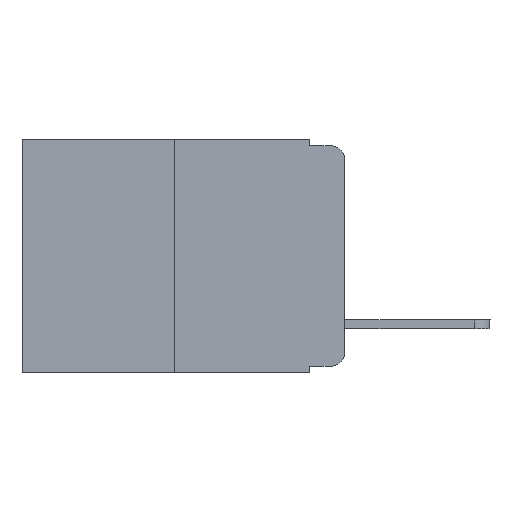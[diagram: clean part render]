
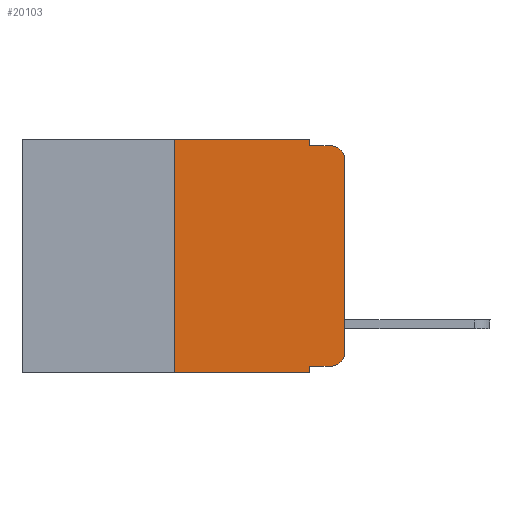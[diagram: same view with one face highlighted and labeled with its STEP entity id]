
A CAD part, left-side view. The second image highlights one B-rep face of the part: STEP entity #20103.
In plain terms, the highlighted planar face has unit normal (-1, 0, 0).
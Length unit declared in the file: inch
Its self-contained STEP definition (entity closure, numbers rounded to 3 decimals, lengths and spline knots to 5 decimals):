
#140 = LINE ( 'NONE', #18347, #10421 ) ;
#152 = CARTESIAN_POINT ( 'NONE',  ( 0., 0.02, -0.03 ) ) ;
#182 = DIRECTION ( 'NONE',  ( 0., 0., -1. ) ) ;
#248 = CARTESIAN_POINT ( 'NONE',  ( 0., 0.051, -0.01 ) ) ;
#279 = DIRECTION ( 'NONE',  ( -1., 0., 0. ) ) ;
#681 = CARTESIAN_POINT ( 'NONE',  ( 0., 0.473, 0. ) ) ;
#867 = CARTESIAN_POINT ( 'NONE',  ( 0., 0.25, 0. ) ) ;
#1016 = ORIENTED_EDGE ( 'NONE', *, *, #3473, .F. ) ;
#1071 = LINE ( 'NONE', #19877, #15737 ) ;
#1551 = VERTEX_POINT ( 'NONE', #14561 ) ;
#1829 = CARTESIAN_POINT ( 'NONE',  ( 0., 0.051, -0.333 ) ) ;
#1869 = CARTESIAN_POINT ( 'NONE',  ( 0., 0.473, 0. ) ) ;
#2087 = ORIENTED_EDGE ( 'NONE', *, *, #14622, .F. ) ;
#2217 = EDGE_CURVE ( 'NONE', #9313, #13193, #4436, .T. ) ;
#2936 = CARTESIAN_POINT ( 'NONE',  ( 0., 0.02, -0.333 ) ) ;
#3215 = EDGE_CURVE ( 'NONE', #13193, #9552, #12734, .T. ) ;
#3347 = ORIENTED_EDGE ( 'NONE', *, *, #13054, .T. ) ;
#3473 = EDGE_CURVE ( 'NONE', #4824, #15468, #13458, .T. ) ;
#3621 = CARTESIAN_POINT ( 'NONE',  ( 0., 0.02, -0.313 ) ) ;
#3670 = EDGE_CURVE ( 'NONE', #12644, #16609, #20081, .T. ) ;
#3690 = VECTOR ( 'NONE', #16941, 39.37008 ) ;
#3915 = DIRECTION ( 'NONE',  ( 0., -1., 0. ) ) ;
#4436 = LINE ( 'NONE', #9757, #4672 ) ;
#4672 = VECTOR ( 'NONE', #5093, 39.37008 ) ;
#4824 = VERTEX_POINT ( 'NONE', #12266 ) ;
#5093 = DIRECTION ( 'NONE',  ( 0., 0., 1. ) ) ;
#5144 = EDGE_CURVE ( 'NONE', #15468, #12644, #16771, .T. ) ;
#5158 = VECTOR ( 'NONE', #7174, 39.37008 ) ;
#5213 = ORIENTED_EDGE ( 'NONE', *, *, #19578, .T. ) ;
#5275 = CARTESIAN_POINT ( 'NONE',  ( 0., 0.051, 0. ) ) ;
#6355 = CARTESIAN_POINT ( 'NONE',  ( 0., 0.25, 0. ) ) ;
#6847 = DIRECTION ( 'NONE',  ( -1., 0., 0. ) ) ;
#7174 = DIRECTION ( 'NONE',  ( 0., 0., 1. ) ) ;
#7466 = AXIS2_PLACEMENT_3D ( 'NONE', #152, #279, #14083 ) ;
#7912 = EDGE_LOOP ( 'NONE', ( #14731, #11924, #2087, #19019, #18644, #1016, #3347, #11121, #12027, #5213 ) ) ;
#8229 = DIRECTION ( 'NONE',  ( 0., 0., -1. ) ) ;
#8286 = CARTESIAN_POINT ( 'NONE',  ( 0., 0., -0.03 ) ) ;
#8431 = DIRECTION ( 'NONE',  ( 0., 0., -1. ) ) ;
#8973 = EDGE_CURVE ( 'NONE', #14886, #1551, #1071, .T. ) ;
#9075 = VECTOR ( 'NONE', #8229, 39.37008 ) ;
#9313 = VERTEX_POINT ( 'NONE', #17843 ) ;
#9552 = VERTEX_POINT ( 'NONE', #12192 ) ;
#9757 = CARTESIAN_POINT ( 'NONE',  ( 0., 0., 0. ) ) ;
#10068 = CARTESIAN_POINT ( 'NONE',  ( 0., 0.473, -0.343 ) ) ;
#10421 = VECTOR ( 'NONE', #13633, 39.37008 ) ;
#11082 = DIRECTION ( 'NONE',  ( 1., 0., 0. ) ) ;
#11121 = ORIENTED_EDGE ( 'NONE', *, *, #8973, .F. ) ;
#11341 = PLANE ( 'NONE',  #18664 ) ;
#11692 = DIRECTION ( 'NONE',  ( 0., -1., 0. ) ) ;
#11825 = VERTEX_POINT ( 'NONE', #2936 ) ;
#11924 = ORIENTED_EDGE ( 'NONE', *, *, #3215, .T. ) ;
#12027 = ORIENTED_EDGE ( 'NONE', *, *, #12214, .T. ) ;
#12089 = DIRECTION ( 'NONE',  ( 0., 0., -1. ) ) ;
#12192 = CARTESIAN_POINT ( 'NONE',  ( 0., 0.02, -0.01 ) ) ;
#12214 = EDGE_CURVE ( 'NONE', #14886, #11825, #140, .T. ) ;
#12266 = CARTESIAN_POINT ( 'NONE',  ( 0., 0.25, -0.343 ) ) ;
#12644 = VERTEX_POINT ( 'NONE', #15055 ) ;
#12734 = CIRCLE ( 'NONE', #7466, 0.02 ) ;
#13054 = EDGE_CURVE ( 'NONE', #4824, #1551, #19146, .T. ) ;
#13193 = VERTEX_POINT ( 'NONE', #8286 ) ;
#13395 = CIRCLE ( 'NONE', #14715, 0.02 ) ;
#13458 = LINE ( 'NONE', #867, #5158 ) ;
#13624 = FACE_OUTER_BOUND ( 'NONE', #7912, .T. ) ;
#13633 = DIRECTION ( 'NONE',  ( 0., -1., 0. ) ) ;
#14083 = DIRECTION ( 'NONE',  ( 0., 0., -1. ) ) ;
#14097 = VECTOR ( 'NONE', #3915, 39.37008 ) ;
#14561 = CARTESIAN_POINT ( 'NONE',  ( 0., 0.051, -0.343 ) ) ;
#14622 = EDGE_CURVE ( 'NONE', #16609, #9552, #14688, .T. ) ;
#14688 = LINE ( 'NONE', #19856, #3690 ) ;
#14715 = AXIS2_PLACEMENT_3D ( 'NONE', #3621, #6847, #8431 ) ;
#14731 = ORIENTED_EDGE ( 'NONE', *, *, #2217, .T. ) ;
#14886 = VERTEX_POINT ( 'NONE', #1829 ) ;
#15055 = CARTESIAN_POINT ( 'NONE',  ( 0., 0.051, 0. ) ) ;
#15468 = VERTEX_POINT ( 'NONE', #6355 ) ;
#15737 = VECTOR ( 'NONE', #12089, 39.37008 ) ;
#16609 = VERTEX_POINT ( 'NONE', #248 ) ;
#16771 = LINE ( 'NONE', #681, #14097 ) ;
#16941 = DIRECTION ( 'NONE',  ( 0., -1., 0. ) ) ;
#17843 = CARTESIAN_POINT ( 'NONE',  ( 0., 0., -0.313 ) ) ;
#18347 = CARTESIAN_POINT ( 'NONE',  ( 0., 0.051, -0.333 ) ) ;
#18644 = ORIENTED_EDGE ( 'NONE', *, *, #5144, .F. ) ;
#18664 = AXIS2_PLACEMENT_3D ( 'NONE', #1869, #11082, #182 ) ;
#19019 = ORIENTED_EDGE ( 'NONE', *, *, #3670, .F. ) ;
#19146 = LINE ( 'NONE', #10068, #19928 ) ;
#19578 = EDGE_CURVE ( 'NONE', #11825, #9313, #13395, .T. ) ;
#19856 = CARTESIAN_POINT ( 'NONE',  ( 0., 0.051, -0.01 ) ) ;
#19877 = CARTESIAN_POINT ( 'NONE',  ( 0., 0.051, 0. ) ) ;
#19928 = VECTOR ( 'NONE', #11692, 39.37008 ) ;
#20081 = LINE ( 'NONE', #5275, #9075 ) ;
#20103 = ADVANCED_FACE ( 'NONE', ( #13624 ), #11341, .F. ) ;
